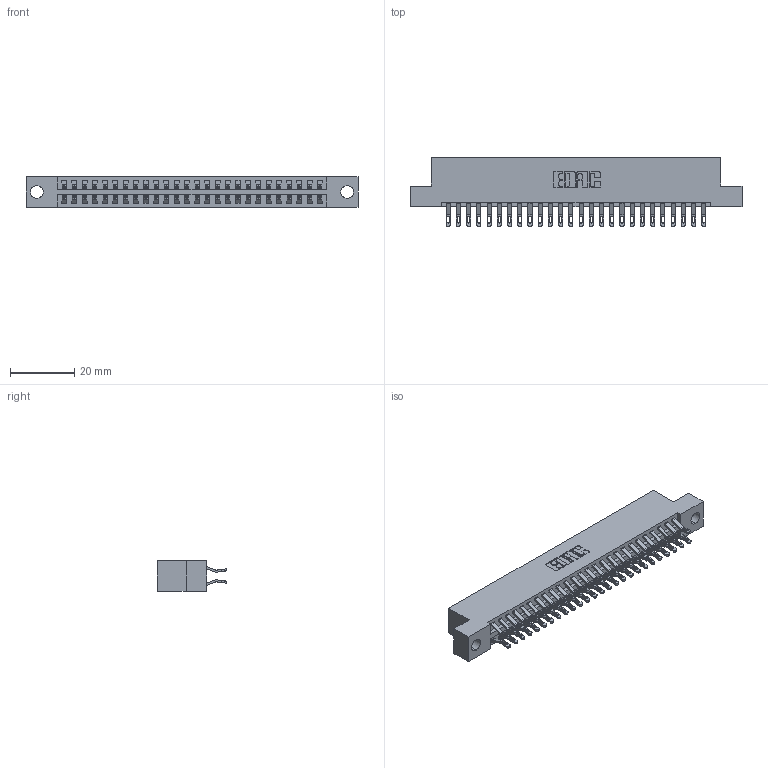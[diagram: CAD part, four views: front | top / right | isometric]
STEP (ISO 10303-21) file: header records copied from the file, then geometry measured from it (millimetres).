
FILE_DESCRIPTION (( 'STEP AP203' ), '1' );
FILE_NAME ('346-052-555-204.STEP', '2022-05-21T01:35:17', ( '' ), ( '' ), 'SwSTEP 2.0', 'SolidWorks 2020', '' );
FILE_SCHEMA (( 'CONFIG_CONTROL_DESIGN' ));
Length unit declared in the file: inch
Products named in the file (3): 345-292-001_555 Tail; 346 Part_Flush Mounting Lugs - 0.156 Dia-TH; 346-052-555-204
Assembly tree (53 placements, depth 2):
  346-052-555-204
    346 Part_Flush Mounting Lugs - 0.156 Dia-TH
    345-292-001_555 Tail  x52
Bounding box: 103.12 x 21.46 x 9.4 mm (x, y, z)
Volume: 9976.5 mm3; surface area: 13847.4 mm2
Topology: 53 solids, 53 shells, 3152 faces, 9881 edges, 6586 vertices
Faces by surface type: plane 1806, cylinder 1346
Entity records: 19867 total; most frequent: CARTESIAN_POINT 3336, ORIENTED_EDGE 3238, DIRECTION 2959, EDGE_CURVE 1619, VECTOR 1363, LINE 1363, VERTEX_POINT 1078, AXIS2_PLACEMENT_3D 798
